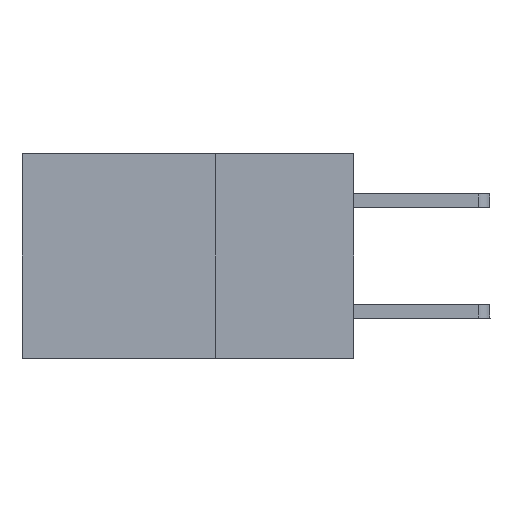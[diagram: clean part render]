
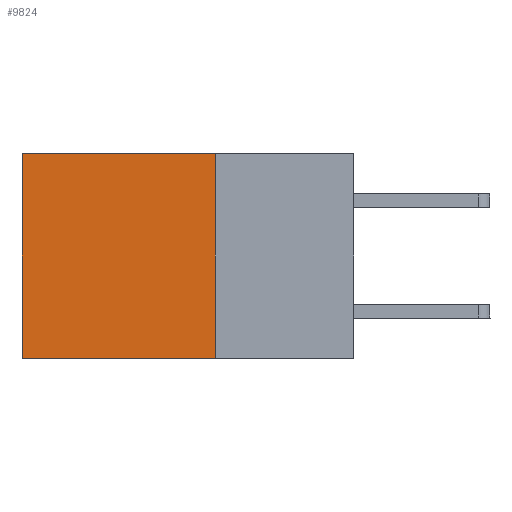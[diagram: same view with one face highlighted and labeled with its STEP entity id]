
A CAD part, left-side view. The second image highlights one B-rep face of the part: STEP entity #9824.
In plain terms, the highlighted planar face has unit normal (-1, 0, 0).
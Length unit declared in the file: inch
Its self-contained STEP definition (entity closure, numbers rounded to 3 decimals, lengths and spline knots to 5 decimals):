
#169 = CARTESIAN_POINT ( 'NONE',  ( 0.2875, 0.6, -0.37 ) ) ;
#351 = CARTESIAN_POINT ( 'NONE',  ( 0.2875, 0.6, 0. ) ) ;
#811 = DIRECTION ( 'NONE',  ( 0., 1., 0. ) ) ;
#1812 = DIRECTION ( 'NONE',  ( 0., 0., -1. ) ) ;
#1842 = CARTESIAN_POINT ( 'NONE',  ( 0.2875, 0.6, 0. ) ) ;
#1884 = LINE ( 'NONE', #10306, #8965 ) ;
#2061 = EDGE_CURVE ( 'NONE', #6687, #11466, #12356, .T. ) ;
#2273 = DIRECTION ( 'NONE',  ( 1., 0., 0. ) ) ;
#2461 = ORIENTED_EDGE ( 'NONE', *, *, #2502, .F. ) ;
#2502 = EDGE_CURVE ( 'NONE', #3840, #11466, #1884, .T. ) ;
#2743 = EDGE_LOOP ( 'NONE', ( #7642, #2461, #3062, #3707 ) ) ;
#3062 = ORIENTED_EDGE ( 'NONE', *, *, #3992, .F. ) ;
#3527 = LINE ( 'NONE', #12138, #7566 ) ;
#3707 = ORIENTED_EDGE ( 'NONE', *, *, #4292, .T. ) ;
#3840 = VERTEX_POINT ( 'NONE', #9238 ) ;
#3992 = EDGE_CURVE ( 'NONE', #8108, #3840, #9606, .T. ) ;
#4292 = EDGE_CURVE ( 'NONE', #8108, #6687, #3527, .T. ) ;
#5992 = CARTESIAN_POINT ( 'NONE',  ( 0.2875, 0.25, 0. ) ) ;
#6009 = CARTESIAN_POINT ( 'NONE',  ( 0.2875, 0.25, 0. ) ) ;
#6056 = DIRECTION ( 'NONE',  ( 0., 0., -1. ) ) ;
#6129 = PLANE ( 'NONE',  #11481 ) ;
#6249 = DIRECTION ( 'NONE',  ( 0., 1., 0. ) ) ;
#6687 = VERTEX_POINT ( 'NONE', #351 ) ;
#7149 = FACE_OUTER_BOUND ( 'NONE', #2743, .T. ) ;
#7566 = VECTOR ( 'NONE', #6249, 39.37008 ) ;
#7642 = ORIENTED_EDGE ( 'NONE', *, *, #2061, .T. ) ;
#8108 = VERTEX_POINT ( 'NONE', #9170 ) ;
#8958 = VECTOR ( 'NONE', #1812, 39.37008 ) ;
#8965 = VECTOR ( 'NONE', #811, 39.37008 ) ;
#9170 = CARTESIAN_POINT ( 'NONE',  ( 0.2875, 0.25, 0. ) ) ;
#9238 = CARTESIAN_POINT ( 'NONE',  ( 0.2875, 0.25, -0.37 ) ) ;
#9606 = LINE ( 'NONE', #5992, #10385 ) ;
#9824 = ADVANCED_FACE ( 'NONE', ( #7149 ), #6129, .F. ) ;
#9997 = DIRECTION ( 'NONE',  ( 0., 0., -1. ) ) ;
#10306 = CARTESIAN_POINT ( 'NONE',  ( 0.2875, 0.25, -0.37 ) ) ;
#10385 = VECTOR ( 'NONE', #6056, 39.37008 ) ;
#11466 = VERTEX_POINT ( 'NONE', #169 ) ;
#11481 = AXIS2_PLACEMENT_3D ( 'NONE', #6009, #2273, #9997 ) ;
#12138 = CARTESIAN_POINT ( 'NONE',  ( 0.2875, 0.25, 0. ) ) ;
#12356 = LINE ( 'NONE', #1842, #8958 ) ;
